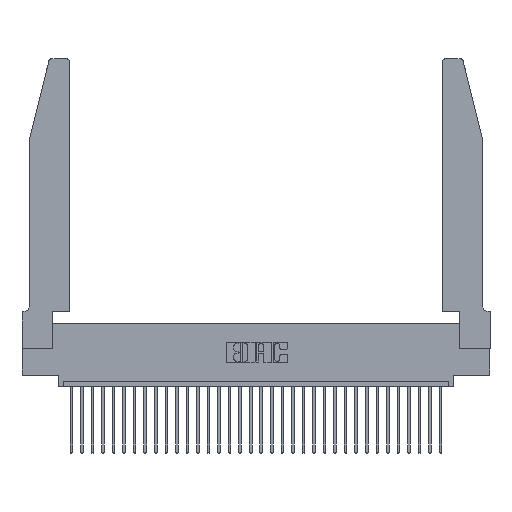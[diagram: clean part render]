
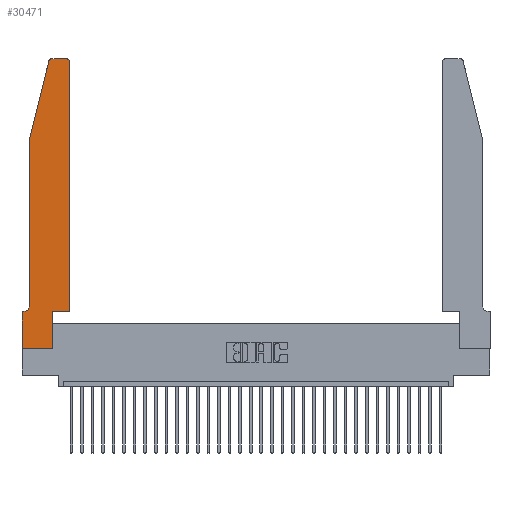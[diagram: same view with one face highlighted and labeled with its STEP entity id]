
A CAD part, top view. The second image highlights one B-rep face of the part: STEP entity #30471.
In plain terms, the highlighted planar face has unit normal (0, 0, 1).
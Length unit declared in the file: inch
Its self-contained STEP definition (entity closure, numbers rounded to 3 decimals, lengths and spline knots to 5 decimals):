
#88 = VERTEX_POINT ( 'NONE', #26625 ) ;
#1147 = CARTESIAN_POINT ( 'NONE',  ( 0.0755, 2., 0.37 ) ) ;
#1236 = LINE ( 'NONE', #13310, #14770 ) ;
#1929 = AXIS2_PLACEMENT_3D ( 'NONE', #27802, #10234, #18051 ) ;
#1973 = CARTESIAN_POINT ( 'NONE',  ( 0.4505, 0.35, 0.37 ) ) ;
#2358 = VERTEX_POINT ( 'NONE', #10709 ) ;
#2495 = DIRECTION ( 'NONE',  ( 0., 1., 0. ) ) ;
#2910 = ORIENTED_EDGE ( 'NONE', *, *, #31317, .T. ) ;
#2997 = VERTEX_POINT ( 'NONE', #8303 ) ;
#3086 = DIRECTION ( 'NONE',  ( -1., 0., 0. ) ) ;
#3190 = LINE ( 'NONE', #23705, #7998 ) ;
#3328 = CARTESIAN_POINT ( 'NONE',  ( 0.0755, 2., 0.37 ) ) ;
#3441 = VERTEX_POINT ( 'NONE', #18348 ) ;
#3761 = AXIS2_PLACEMENT_3D ( 'NONE', #4718, #27559, #24612 ) ;
#3939 = VECTOR ( 'NONE', #5813, 39.37008 ) ;
#4548 = EDGE_CURVE ( 'NONE', #15278, #3441, #15524, .T. ) ;
#4718 = CARTESIAN_POINT ( 'NONE',  ( 0.284, 2.72, 0.37 ) ) ;
#5016 = DIRECTION ( 'NONE',  ( -1., 0., 0. ) ) ;
#5449 = VERTEX_POINT ( 'NONE', #10894 ) ;
#5813 = DIRECTION ( 'NONE',  ( -1., 0., 0. ) ) ;
#5819 = DIRECTION ( 'NONE',  ( 0., 0., 1. ) ) ;
#6239 = DIRECTION ( 'NONE',  ( 0., -1., 0. ) ) ;
#6424 = CARTESIAN_POINT ( 'NONE',  ( 0., 0.35, 0.37 ) ) ;
#6532 = CIRCLE ( 'NONE', #1929, 0.03 ) ;
#6868 = VECTOR ( 'NONE', #26390, 39.37008 ) ;
#6974 = EDGE_CURVE ( 'NONE', #5449, #88, #26787, .T. ) ;
#7256 = ORIENTED_EDGE ( 'NONE', *, *, #6974, .T. ) ;
#7660 = EDGE_CURVE ( 'NONE', #13917, #5449, #8514, .T. ) ;
#7970 = EDGE_CURVE ( 'NONE', #17819, #2997, #16485, .T. ) ;
#7998 = VECTOR ( 'NONE', #3086, 39.37008 ) ;
#8303 = CARTESIAN_POINT ( 'NONE',  ( 0.25487, 2.72718, 0.37 ) ) ;
#8514 = LINE ( 'NONE', #26380, #20053 ) ;
#10234 = DIRECTION ( 'NONE',  ( 0., 0., 1. ) ) ;
#10287 = CARTESIAN_POINT ( 'NONE',  ( 0., 0., 0.37 ) ) ;
#10565 = VERTEX_POINT ( 'NONE', #14042 ) ;
#10578 = VECTOR ( 'NONE', #30672, 39.37008 ) ;
#10709 = CARTESIAN_POINT ( 'NONE',  ( 0.0755, 0.42, 0.37 ) ) ;
#10894 = CARTESIAN_POINT ( 'NONE',  ( 0., 0., 0.37 ) ) ;
#11184 = PLANE ( 'NONE',  #23906 ) ;
#11201 = ORIENTED_EDGE ( 'NONE', *, *, #27686, .T. ) ;
#11377 = CARTESIAN_POINT ( 'NONE',  ( 0.284, 2.75, 0.37 ) ) ;
#11427 = EDGE_CURVE ( 'NONE', #2997, #12098, #18350, .T. ) ;
#11439 = CARTESIAN_POINT ( 'NONE',  ( 0.0055, 0.35, 0.37 ) ) ;
#11757 = EDGE_CURVE ( 'NONE', #88, #15278, #27020, .T. ) ;
#11831 = EDGE_CURVE ( 'NONE', #10565, #17819, #3190, .T. ) ;
#12098 = VERTEX_POINT ( 'NONE', #1147 ) ;
#12251 = ORIENTED_EDGE ( 'NONE', *, *, #11831, .T. ) ;
#12292 = CARTESIAN_POINT ( 'NONE',  ( 0.0055, 0.42, 0.37 ) ) ;
#13310 = CARTESIAN_POINT ( 'NONE',  ( 0.0755, 2., 0.37 ) ) ;
#13917 = VERTEX_POINT ( 'NONE', #6424 ) ;
#14042 = CARTESIAN_POINT ( 'NONE',  ( 0.4205, 2.75, 0.37 ) ) ;
#14066 = ORIENTED_EDGE ( 'NONE', *, *, #7970, .T. ) ;
#14324 = LINE ( 'NONE', #24906, #3939 ) ;
#14537 = DIRECTION ( 'NONE',  ( 0., -1., 0. ) ) ;
#14770 = VECTOR ( 'NONE', #14537, 39.37008 ) ;
#15278 = VERTEX_POINT ( 'NONE', #25917 ) ;
#15524 = LINE ( 'NONE', #1973, #26980 ) ;
#15756 = ORIENTED_EDGE ( 'NONE', *, *, #11427, .T. ) ;
#16485 = CIRCLE ( 'NONE', #3761, 0.03 ) ;
#16778 = ORIENTED_EDGE ( 'NONE', *, *, #25077, .T. ) ;
#16925 = EDGE_CURVE ( 'NONE', #12098, #2358, #1236, .T. ) ;
#17574 = DIRECTION ( 'NONE',  ( 0., 0., -1. ) ) ;
#17819 = VERTEX_POINT ( 'NONE', #11377 ) ;
#18049 = CARTESIAN_POINT ( 'NONE',  ( 0.4505, 0.35, 0.37 ) ) ;
#18051 = DIRECTION ( 'NONE',  ( 1., 0., 0. ) ) ;
#18169 = CIRCLE ( 'NONE', #20738, 0.07 ) ;
#18348 = CARTESIAN_POINT ( 'NONE',  ( 0.4505, 0.35, 0.37 ) ) ;
#18350 = LINE ( 'NONE', #3328, #6868 ) ;
#19420 = CARTESIAN_POINT ( 'NONE',  ( 0.4505, 2.72, 0.37 ) ) ;
#20053 = VECTOR ( 'NONE', #6239, 39.37008 ) ;
#20182 = EDGE_CURVE ( 'NONE', #27640, #13917, #14324, .T. ) ;
#20530 = ORIENTED_EDGE ( 'NONE', *, *, #7660, .T. ) ;
#20738 = AXIS2_PLACEMENT_3D ( 'NONE', #12292, #17574, #5016 ) ;
#20984 = CARTESIAN_POINT ( 'NONE',  ( 0., 0.35, 0.37 ) ) ;
#23360 = ORIENTED_EDGE ( 'NONE', *, *, #20182, .T. ) ;
#23454 = VECTOR ( 'NONE', #2495, 39.37008 ) ;
#23555 = DIRECTION ( 'NONE',  ( 1., 0., 0. ) ) ;
#23705 = CARTESIAN_POINT ( 'NONE',  ( 0.2605, 2.75, 0.37 ) ) ;
#23906 = AXIS2_PLACEMENT_3D ( 'NONE', #20984, #5819, #23555 ) ;
#24573 = DIRECTION ( 'NONE',  ( 1., 0., 0. ) ) ;
#24612 = DIRECTION ( 'NONE',  ( 1., 0., 0. ) ) ;
#24811 = ORIENTED_EDGE ( 'NONE', *, *, #4548, .T. ) ;
#24906 = CARTESIAN_POINT ( 'NONE',  ( 0.0755, 0.35, 0.37 ) ) ;
#25077 = EDGE_CURVE ( 'NONE', #31789, #10565, #6532, .T. ) ;
#25278 = EDGE_LOOP ( 'NONE', ( #12251, #14066, #15756, #30074, #2910, #23360, #20530, #7256, #28061, #24811, #11201, #16778 ) ) ;
#25344 = VECTOR ( 'NONE', #30414, 39.37008 ) ;
#25917 = CARTESIAN_POINT ( 'NONE',  ( 0.2865, 0.35, 0.37 ) ) ;
#26380 = CARTESIAN_POINT ( 'NONE',  ( 0., 0., 0.37 ) ) ;
#26390 = DIRECTION ( 'NONE',  ( -0.239, -0.971, 0. ) ) ;
#26625 = CARTESIAN_POINT ( 'NONE',  ( 0.2865, 0., 0.37 ) ) ;
#26787 = LINE ( 'NONE', #10287, #10578 ) ;
#26980 = VECTOR ( 'NONE', #24573, 39.37008 ) ;
#27020 = LINE ( 'NONE', #30516, #23454 ) ;
#27559 = DIRECTION ( 'NONE',  ( 0., 0., 1. ) ) ;
#27640 = VERTEX_POINT ( 'NONE', #11439 ) ;
#27686 = EDGE_CURVE ( 'NONE', #3441, #31789, #32082, .T. ) ;
#27802 = CARTESIAN_POINT ( 'NONE',  ( 0.4205, 2.72, 0.37 ) ) ;
#28061 = ORIENTED_EDGE ( 'NONE', *, *, #11757, .T. ) ;
#29685 = FACE_OUTER_BOUND ( 'NONE', #25278, .T. ) ;
#30074 = ORIENTED_EDGE ( 'NONE', *, *, #16925, .T. ) ;
#30414 = DIRECTION ( 'NONE',  ( 0., 1., 0. ) ) ;
#30471 = ADVANCED_FACE ( 'NONE', ( #29685 ), #11184, .T. ) ;
#30516 = CARTESIAN_POINT ( 'NONE',  ( 0.2865, 0.35, 0.37 ) ) ;
#30672 = DIRECTION ( 'NONE',  ( 1., 0., 0. ) ) ;
#31317 = EDGE_CURVE ( 'NONE', #2358, #27640, #18169, .T. ) ;
#31789 = VERTEX_POINT ( 'NONE', #19420 ) ;
#32082 = LINE ( 'NONE', #18049, #25344 ) ;
